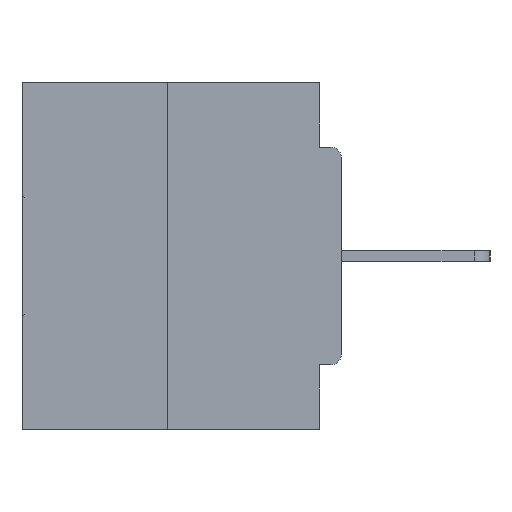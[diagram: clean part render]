
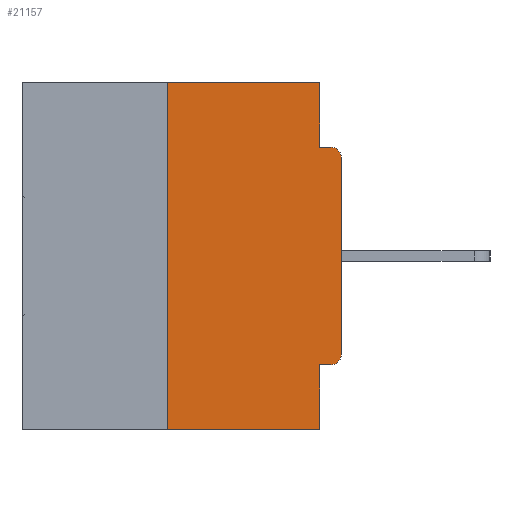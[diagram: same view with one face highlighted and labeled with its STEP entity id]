
A CAD part, left-side view. The second image highlights one B-rep face of the part: STEP entity #21157.
In plain terms, the highlighted planar face has unit normal (-1, 0, 0).
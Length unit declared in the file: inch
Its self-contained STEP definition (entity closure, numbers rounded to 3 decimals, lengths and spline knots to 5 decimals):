
#37 = CARTESIAN_POINT ( 'NONE',  ( 0., 0.25, 0. ) ) ;
#74 = DIRECTION ( 'NONE',  ( -1., 0., 0. ) ) ;
#811 = CIRCLE ( 'NONE', #20883, 0.015 ) ;
#1236 = VECTOR ( 'NONE', #19153, 39.37008 ) ;
#1392 = AXIS2_PLACEMENT_3D ( 'NONE', #3310, #74, #11033 ) ;
#1583 = CARTESIAN_POINT ( 'NONE',  ( 0., 0.015, -0.3915 ) ) ;
#1603 = ORIENTED_EDGE ( 'NONE', *, *, #31707, .F. ) ;
#1616 = CARTESIAN_POINT ( 'NONE',  ( 0., 0.031, 0. ) ) ;
#2582 = VERTEX_POINT ( 'NONE', #27979 ) ;
#2610 = CARTESIAN_POINT ( 'NONE',  ( 0., 0.46, 0. ) ) ;
#2853 = ORIENTED_EDGE ( 'NONE', *, *, #25845, .F. ) ;
#3099 = ORIENTED_EDGE ( 'NONE', *, *, #7147, .F. ) ;
#3151 = LINE ( 'NONE', #8192, #1236 ) ;
#3286 = LINE ( 'NONE', #25540, #23084 ) ;
#3310 = CARTESIAN_POINT ( 'NONE',  ( 0., 0.015, -0.1085 ) ) ;
#3570 = VERTEX_POINT ( 'NONE', #14672 ) ;
#3862 = CARTESIAN_POINT ( 'NONE',  ( 0., 0.015, -0.4065 ) ) ;
#4086 = ORIENTED_EDGE ( 'NONE', *, *, #35229, .T. ) ;
#4376 = VERTEX_POINT ( 'NONE', #1616 ) ;
#4450 = DIRECTION ( 'NONE',  ( 0., 0., -1. ) ) ;
#4687 = DIRECTION ( 'NONE',  ( 0., 1., 0. ) ) ;
#4836 = CIRCLE ( 'NONE', #1392, 0.015 ) ;
#4925 = VECTOR ( 'NONE', #16544, 39.37008 ) ;
#5227 = CARTESIAN_POINT ( 'NONE',  ( 0., 0.015, -0.0935 ) ) ;
#5430 = CARTESIAN_POINT ( 'NONE',  ( 0., 0.031, -0.4065 ) ) ;
#5440 = DIRECTION ( 'NONE',  ( 0., 0., 1. ) ) ;
#5843 = CARTESIAN_POINT ( 'NONE',  ( 0., 0., -0.3915 ) ) ;
#6214 = ORIENTED_EDGE ( 'NONE', *, *, #32857, .F. ) ;
#6649 = EDGE_CURVE ( 'NONE', #11036, #28071, #4836, .T. ) ;
#7147 = EDGE_CURVE ( 'NONE', #20489, #2582, #30583, .T. ) ;
#8096 = ORIENTED_EDGE ( 'NONE', *, *, #31119, .F. ) ;
#8192 = CARTESIAN_POINT ( 'NONE',  ( 0., 0., -0.0935 ) ) ;
#8234 = CARTESIAN_POINT ( 'NONE',  ( 0., 0.031, -0.5 ) ) ;
#8573 = LINE ( 'NONE', #27824, #10381 ) ;
#10381 = VECTOR ( 'NONE', #22213, 39.37008 ) ;
#10433 = LINE ( 'NONE', #12751, #23901 ) ;
#11033 = DIRECTION ( 'NONE',  ( 0., 0., -1. ) ) ;
#11036 = VERTEX_POINT ( 'NONE', #29361 ) ;
#11847 = ORIENTED_EDGE ( 'NONE', *, *, #34250, .F. ) ;
#12183 = VERTEX_POINT ( 'NONE', #3862 ) ;
#12751 = CARTESIAN_POINT ( 'NONE',  ( 0., 0., -0.4065 ) ) ;
#12888 = VERTEX_POINT ( 'NONE', #5430 ) ;
#13142 = LINE ( 'NONE', #27203, #29259 ) ;
#14672 = CARTESIAN_POINT ( 'NONE',  ( 0., 0.031, -0.0935 ) ) ;
#15731 = VECTOR ( 'NONE', #5440, 39.37008 ) ;
#16544 = DIRECTION ( 'NONE',  ( 0., -1., 0. ) ) ;
#16731 = LINE ( 'NONE', #19253, #4925 ) ;
#18273 = DIRECTION ( 'NONE',  ( -1., 0., 0. ) ) ;
#19153 = DIRECTION ( 'NONE',  ( 0., -1., 0. ) ) ;
#19164 = AXIS2_PLACEMENT_3D ( 'NONE', #34445, #23819, #23285 ) ;
#19253 = CARTESIAN_POINT ( 'NONE',  ( 0., 0.46, -0.5 ) ) ;
#20489 = VERTEX_POINT ( 'NONE', #25157 ) ;
#20883 = AXIS2_PLACEMENT_3D ( 'NONE', #1583, #18273, #4450 ) ;
#21157 = ADVANCED_FACE ( 'NONE', ( #26558 ), #28706, .F. ) ;
#21170 = EDGE_CURVE ( 'NONE', #12183, #31207, #811, .T. ) ;
#22086 = EDGE_LOOP ( 'NONE', ( #8096, #3099, #30561, #6214, #2853, #29357, #4086, #32128, #11847, #1603 ) ) ;
#22213 = DIRECTION ( 'NONE',  ( 0., 0., 1. ) ) ;
#22476 = DIRECTION ( 'NONE',  ( 0., 0., -1. ) ) ;
#23084 = VECTOR ( 'NONE', #22476, 39.37008 ) ;
#23129 = EDGE_CURVE ( 'NONE', #20489, #28553, #16731, .T. ) ;
#23285 = DIRECTION ( 'NONE',  ( 0., 0., -1. ) ) ;
#23819 = DIRECTION ( 'NONE',  ( 1., 0., 0. ) ) ;
#23901 = VECTOR ( 'NONE', #4687, 39.37008 ) ;
#24511 = DIRECTION ( 'NONE',  ( 0., -1., 0. ) ) ;
#24645 = DIRECTION ( 'NONE',  ( 0., 0., -1. ) ) ;
#25157 = CARTESIAN_POINT ( 'NONE',  ( 0., 0.25, -0.5 ) ) ;
#25540 = CARTESIAN_POINT ( 'NONE',  ( 0., 0.031, 0. ) ) ;
#25845 = EDGE_CURVE ( 'NONE', #12183, #12888, #10433, .T. ) ;
#26558 = FACE_OUTER_BOUND ( 'NONE', #22086, .T. ) ;
#27203 = CARTESIAN_POINT ( 'NONE',  ( 0., 0.031, -0.5 ) ) ;
#27824 = CARTESIAN_POINT ( 'NONE',  ( 0., 0., 0. ) ) ;
#27979 = CARTESIAN_POINT ( 'NONE',  ( 0., 0.25, 0. ) ) ;
#28071 = VERTEX_POINT ( 'NONE', #5227 ) ;
#28553 = VERTEX_POINT ( 'NONE', #8234 ) ;
#28706 = PLANE ( 'NONE',  #19164 ) ;
#29259 = VECTOR ( 'NONE', #24645, 39.37008 ) ;
#29357 = ORIENTED_EDGE ( 'NONE', *, *, #21170, .T. ) ;
#29361 = CARTESIAN_POINT ( 'NONE',  ( 0., 0., -0.1085 ) ) ;
#29923 = LINE ( 'NONE', #2610, #29965 ) ;
#29965 = VECTOR ( 'NONE', #24511, 39.37008 ) ;
#30561 = ORIENTED_EDGE ( 'NONE', *, *, #23129, .T. ) ;
#30583 = LINE ( 'NONE', #37, #15731 ) ;
#31119 = EDGE_CURVE ( 'NONE', #2582, #4376, #29923, .T. ) ;
#31207 = VERTEX_POINT ( 'NONE', #5843 ) ;
#31707 = EDGE_CURVE ( 'NONE', #4376, #3570, #3286, .T. ) ;
#32128 = ORIENTED_EDGE ( 'NONE', *, *, #6649, .T. ) ;
#32857 = EDGE_CURVE ( 'NONE', #12888, #28553, #13142, .T. ) ;
#34250 = EDGE_CURVE ( 'NONE', #3570, #28071, #3151, .T. ) ;
#34445 = CARTESIAN_POINT ( 'NONE',  ( 0., 0.46, 0. ) ) ;
#35229 = EDGE_CURVE ( 'NONE', #31207, #11036, #8573, .T. ) ;
